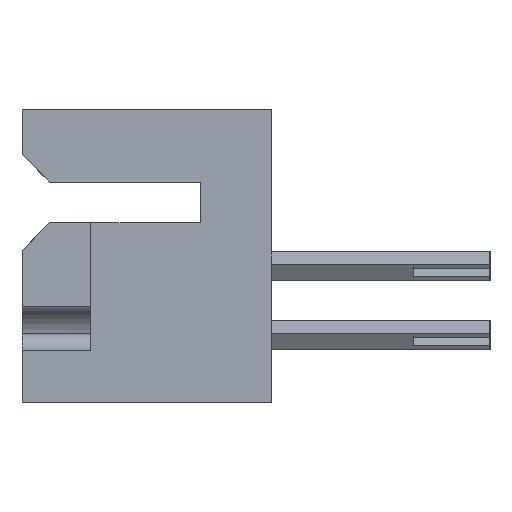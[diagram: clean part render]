
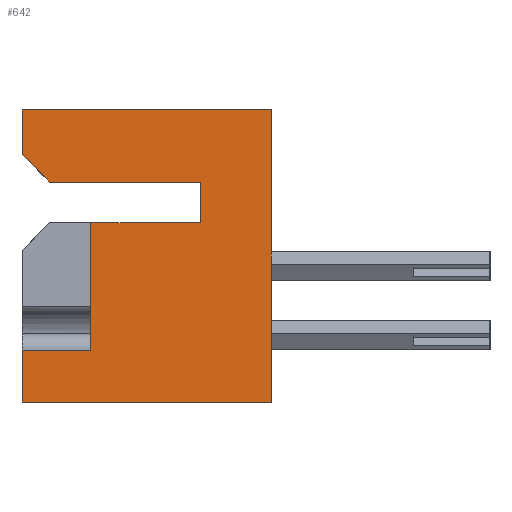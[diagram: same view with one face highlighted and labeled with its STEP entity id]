
A CAD part, left-side view. The second image highlights one B-rep face of the part: STEP entity #642.
In plain terms, the highlighted planar face has unit normal (-1, 0, 0).
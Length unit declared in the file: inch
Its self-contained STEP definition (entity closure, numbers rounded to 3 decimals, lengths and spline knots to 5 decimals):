
#109 = VERTEX_POINT ( 'NONE', #16499 ) ;
#548 = DIRECTION ( 'NONE',  ( 0., 1., 0. ) ) ;
#573 = EDGE_CURVE ( 'NONE', #6778, #109, #13594, .T. ) ;
#626 = DIRECTION ( 'NONE',  ( 0., 0., 1. ) ) ;
#637 = LINE ( 'NONE', #754, #7877 ) ;
#642 = ADVANCED_FACE ( 'NONE', ( #18670 ), #11459, .F. ) ;
#754 = CARTESIAN_POINT ( 'NONE',  ( 0., 0.128, -0.205 ) ) ;
#811 = EDGE_CURVE ( 'NONE', #20056, #10977, #1204, .T. ) ;
#888 = LINE ( 'NONE', #3339, #17066 ) ;
#1204 = LINE ( 'NONE', #13444, #17675 ) ;
#1543 = ORIENTED_EDGE ( 'NONE', *, *, #811, .T. ) ;
#1674 = CARTESIAN_POINT ( 'NONE',  ( 0., 0.128, -0.131 ) ) ;
#1709 = LINE ( 'NONE', #16541, #3460 ) ;
#2085 = DIRECTION ( 'NONE',  ( 0., 0., -1. ) ) ;
#2170 = EDGE_CURVE ( 'NONE', #20056, #6778, #9431, .T. ) ;
#2996 = LINE ( 'NONE', #13584, #19705 ) ;
#3249 = ORIENTED_EDGE ( 'NONE', *, *, #9967, .T. ) ;
#3339 = CARTESIAN_POINT ( 'NONE',  ( 0., 0.453, -0.531 ) ) ;
#3460 = VECTOR ( 'NONE', #20016, 39.37008 ) ;
#3686 = DIRECTION ( 'NONE',  ( 1., 0., 0. ) ) ;
#4134 = CARTESIAN_POINT ( 'NONE',  ( 0., 0.453, 0. ) ) ;
#4157 = DIRECTION ( 'NONE',  ( 0., 0., 1. ) ) ;
#4367 = VERTEX_POINT ( 'NONE', #5010 ) ;
#4844 = ORIENTED_EDGE ( 'NONE', *, *, #6780, .T. ) ;
#4957 = VECTOR ( 'NONE', #19486, 39.37008 ) ;
#4966 = VERTEX_POINT ( 'NONE', #19948 ) ;
#5010 = CARTESIAN_POINT ( 'NONE',  ( 0., 0.453, -0.437 ) ) ;
#5333 = ORIENTED_EDGE ( 'NONE', *, *, #15423, .F. ) ;
#5560 = EDGE_LOOP ( 'NONE', ( #20245, #7518, #6234, #3249, #18960, #17159, #1543, #11993, #17743, #4844, #5333 ) ) ;
#5584 = LINE ( 'NONE', #8437, #18047 ) ;
#5644 = CARTESIAN_POINT ( 'NONE',  ( 0., 0.453, -0.531 ) ) ;
#5894 = EDGE_CURVE ( 'NONE', #20284, #10977, #6385, .T. ) ;
#6234 = ORIENTED_EDGE ( 'NONE', *, *, #6940, .T. ) ;
#6385 = LINE ( 'NONE', #13915, #18101 ) ;
#6407 = CARTESIAN_POINT ( 'NONE',  ( 0., 0.453, 0. ) ) ;
#6692 = VECTOR ( 'NONE', #7637, 39.37008 ) ;
#6778 = VERTEX_POINT ( 'NONE', #8513 ) ;
#6780 = EDGE_CURVE ( 'NONE', #17962, #14487, #637, .T. ) ;
#6903 = VECTOR ( 'NONE', #15384, 39.37008 ) ;
#6940 = EDGE_CURVE ( 'NONE', #19199, #4966, #888, .T. ) ;
#7216 = DIRECTION ( 'NONE',  ( 0., 1., 0. ) ) ;
#7518 = ORIENTED_EDGE ( 'NONE', *, *, #8591, .F. ) ;
#7637 = DIRECTION ( 'NONE',  ( 0., 0., 1. ) ) ;
#7877 = VECTOR ( 'NONE', #548, 39.37008 ) ;
#8437 = CARTESIAN_POINT ( 'NONE',  ( 0., 0.328, -0.205 ) ) ;
#8513 = CARTESIAN_POINT ( 'NONE',  ( 0., 0.453, 0. ) ) ;
#8591 = EDGE_CURVE ( 'NONE', #19199, #4367, #10392, .T. ) ;
#8857 = CARTESIAN_POINT ( 'NONE',  ( 0., 0.453, 0. ) ) ;
#8886 = CARTESIAN_POINT ( 'NONE',  ( 0., 0.128, -0.205 ) ) ;
#8899 = AXIS2_PLACEMENT_3D ( 'NONE', #11521, #3686, #2085 ) ;
#9333 = VECTOR ( 'NONE', #4157, 39.37008 ) ;
#9431 = LINE ( 'NONE', #4134, #6903 ) ;
#9788 = DIRECTION ( 'NONE',  ( 0., -1., 0. ) ) ;
#9967 = EDGE_CURVE ( 'NONE', #4966, #109, #19414, .T. ) ;
#10392 = LINE ( 'NONE', #8857, #9333 ) ;
#10977 = VERTEX_POINT ( 'NONE', #11290 ) ;
#11290 = CARTESIAN_POINT ( 'NONE',  ( 0., 0.403, -0.131 ) ) ;
#11459 = PLANE ( 'NONE',  #8899 ) ;
#11521 = CARTESIAN_POINT ( 'NONE',  ( 0., 0.453, 0. ) ) ;
#11993 = ORIENTED_EDGE ( 'NONE', *, *, #5894, .F. ) ;
#12112 = CARTESIAN_POINT ( 'NONE',  ( 0., 0.453, -0.081 ) ) ;
#12466 = CARTESIAN_POINT ( 'NONE',  ( 0., 0.328, -0.205 ) ) ;
#13444 = CARTESIAN_POINT ( 'NONE',  ( 0., 0.403, -0.131 ) ) ;
#13584 = CARTESIAN_POINT ( 'NONE',  ( 0., 0.128, -0.131 ) ) ;
#13594 = LINE ( 'NONE', #6407, #4957 ) ;
#13848 = CARTESIAN_POINT ( 'NONE',  ( 0., 0., 0. ) ) ;
#13915 = CARTESIAN_POINT ( 'NONE',  ( 0., 0.128, -0.131 ) ) ;
#14487 = VERTEX_POINT ( 'NONE', #12466 ) ;
#14852 = DIRECTION ( 'NONE',  ( 0., 0., 1. ) ) ;
#15384 = DIRECTION ( 'NONE',  ( 0., 0., 1. ) ) ;
#15423 = EDGE_CURVE ( 'NONE', #17472, #14487, #5584, .T. ) ;
#16499 = CARTESIAN_POINT ( 'NONE',  ( 0., 0., 0. ) ) ;
#16541 = CARTESIAN_POINT ( 'NONE',  ( 0., 0.328, -0.437 ) ) ;
#16699 = EDGE_CURVE ( 'NONE', #17962, #20284, #2996, .T. ) ;
#17066 = VECTOR ( 'NONE', #9788, 39.37008 ) ;
#17159 = ORIENTED_EDGE ( 'NONE', *, *, #2170, .F. ) ;
#17239 = EDGE_CURVE ( 'NONE', #17472, #4367, #1709, .T. ) ;
#17472 = VERTEX_POINT ( 'NONE', #20364 ) ;
#17675 = VECTOR ( 'NONE', #18404, 39.37008 ) ;
#17743 = ORIENTED_EDGE ( 'NONE', *, *, #16699, .F. ) ;
#17962 = VERTEX_POINT ( 'NONE', #8886 ) ;
#18047 = VECTOR ( 'NONE', #14852, 39.37008 ) ;
#18101 = VECTOR ( 'NONE', #7216, 39.37008 ) ;
#18404 = DIRECTION ( 'NONE',  ( 0., -0.707, -0.707 ) ) ;
#18670 = FACE_OUTER_BOUND ( 'NONE', #5560, .T. ) ;
#18960 = ORIENTED_EDGE ( 'NONE', *, *, #573, .F. ) ;
#19199 = VERTEX_POINT ( 'NONE', #5644 ) ;
#19414 = LINE ( 'NONE', #13848, #6692 ) ;
#19486 = DIRECTION ( 'NONE',  ( 0., -1., 0. ) ) ;
#19705 = VECTOR ( 'NONE', #626, 39.37008 ) ;
#19948 = CARTESIAN_POINT ( 'NONE',  ( 0., 0., -0.531 ) ) ;
#20016 = DIRECTION ( 'NONE',  ( 0., 1., 0. ) ) ;
#20056 = VERTEX_POINT ( 'NONE', #12112 ) ;
#20245 = ORIENTED_EDGE ( 'NONE', *, *, #17239, .T. ) ;
#20284 = VERTEX_POINT ( 'NONE', #1674 ) ;
#20364 = CARTESIAN_POINT ( 'NONE',  ( 0., 0.328, -0.437 ) ) ;
